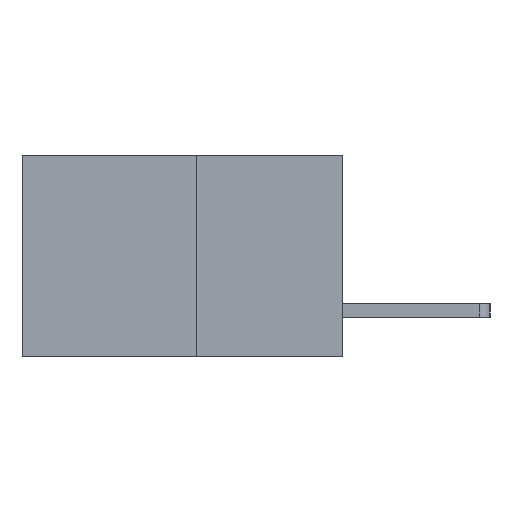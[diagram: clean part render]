
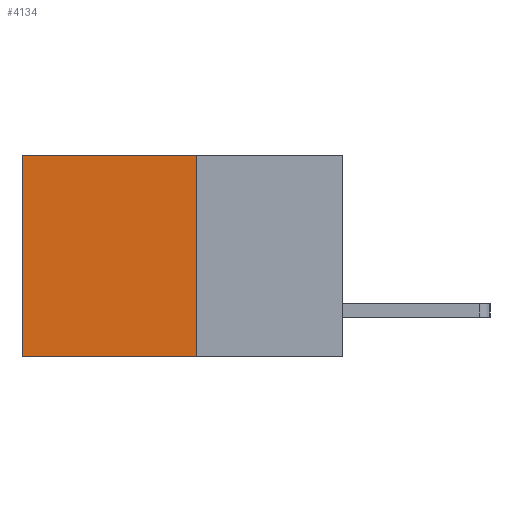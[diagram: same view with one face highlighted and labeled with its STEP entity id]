
A CAD part, left-side view. The second image highlights one B-rep face of the part: STEP entity #4134.
In plain terms, the highlighted planar face has unit normal (-1, 0, 0).
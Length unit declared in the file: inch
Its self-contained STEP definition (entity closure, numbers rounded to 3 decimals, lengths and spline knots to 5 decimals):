
#22 = DIRECTION ( 'NONE',  ( 0., 1., 0. ) ) ;
#207 = EDGE_CURVE ( 'NONE', #1928, #728, #4651, .T. ) ;
#728 = VERTEX_POINT ( 'NONE', #4153 ) ;
#811 = VECTOR ( 'NONE', #5093, 39.37008 ) ;
#1440 = LINE ( 'NONE', #7465, #5809 ) ;
#1696 = ORIENTED_EDGE ( 'NONE', *, *, #207, .F. ) ;
#1928 = VERTEX_POINT ( 'NONE', #5198 ) ;
#2035 = EDGE_CURVE ( 'NONE', #728, #8117, #1440, .T. ) ;
#2273 = LINE ( 'NONE', #6788, #11029 ) ;
#3189 = LINE ( 'NONE', #10140, #811 ) ;
#3225 = EDGE_CURVE ( 'NONE', #1928, #3682, #2273, .T. ) ;
#3682 = VERTEX_POINT ( 'NONE', #4457 ) ;
#3747 = ORIENTED_EDGE ( 'NONE', *, *, #2035, .F. ) ;
#4134 = ADVANCED_FACE ( 'NONE', ( #8433 ), #11006, .F. ) ;
#4153 = CARTESIAN_POINT ( 'NONE',  ( 0.277, 0.27, -0.37 ) ) ;
#4271 = ORIENTED_EDGE ( 'NONE', *, *, #3225, .T. ) ;
#4457 = CARTESIAN_POINT ( 'NONE',  ( 0.277, 0.59, 0. ) ) ;
#4651 = LINE ( 'NONE', #7276, #6990 ) ;
#4933 = ORIENTED_EDGE ( 'NONE', *, *, #8219, .T. ) ;
#5027 = AXIS2_PLACEMENT_3D ( 'NONE', #11140, #10981, #10869 ) ;
#5073 = DIRECTION ( 'NONE',  ( 0., 1., 0. ) ) ;
#5093 = DIRECTION ( 'NONE',  ( 0., 0., -1. ) ) ;
#5198 = CARTESIAN_POINT ( 'NONE',  ( 0.277, 0.27, 0. ) ) ;
#5267 = DIRECTION ( 'NONE',  ( 0., 0., -1. ) ) ;
#5792 = EDGE_LOOP ( 'NONE', ( #4933, #3747, #1696, #4271 ) ) ;
#5809 = VECTOR ( 'NONE', #5073, 39.37008 ) ;
#6788 = CARTESIAN_POINT ( 'NONE',  ( 0.277, 0.27, 0. ) ) ;
#6990 = VECTOR ( 'NONE', #5267, 39.37008 ) ;
#7276 = CARTESIAN_POINT ( 'NONE',  ( 0.277, 0.27, -0.37 ) ) ;
#7465 = CARTESIAN_POINT ( 'NONE',  ( 0.277, 0.27, -0.37 ) ) ;
#8117 = VERTEX_POINT ( 'NONE', #10822 ) ;
#8219 = EDGE_CURVE ( 'NONE', #3682, #8117, #3189, .T. ) ;
#8433 = FACE_OUTER_BOUND ( 'NONE', #5792, .T. ) ;
#10140 = CARTESIAN_POINT ( 'NONE',  ( 0.277, 0.59, -0.37 ) ) ;
#10822 = CARTESIAN_POINT ( 'NONE',  ( 0.277, 0.59, -0.37 ) ) ;
#10869 = DIRECTION ( 'NONE',  ( 0., 0., -1. ) ) ;
#10981 = DIRECTION ( 'NONE',  ( 1., 0., 0. ) ) ;
#11006 = PLANE ( 'NONE',  #5027 ) ;
#11029 = VECTOR ( 'NONE', #22, 39.37008 ) ;
#11140 = CARTESIAN_POINT ( 'NONE',  ( 0.277, 0.27, -0.37 ) ) ;
